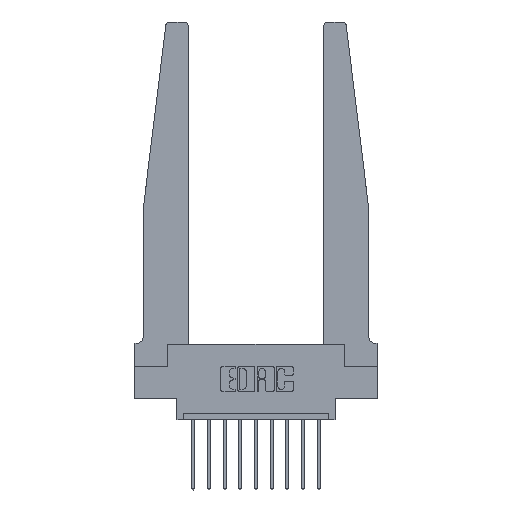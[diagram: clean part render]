
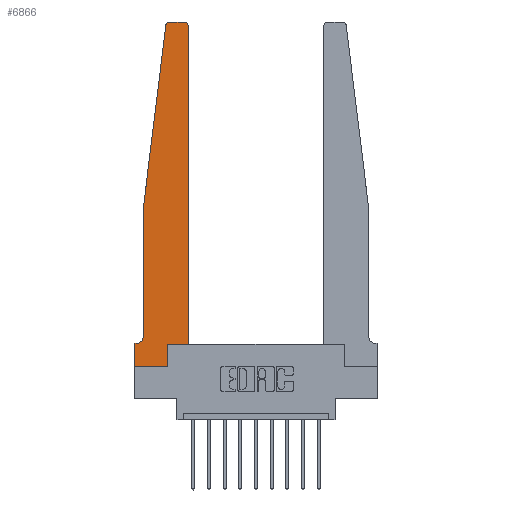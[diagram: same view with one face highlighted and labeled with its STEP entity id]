
A CAD part, top view. The second image highlights one B-rep face of the part: STEP entity #6866.
In plain terms, the highlighted planar face has unit normal (0, 0, 1).
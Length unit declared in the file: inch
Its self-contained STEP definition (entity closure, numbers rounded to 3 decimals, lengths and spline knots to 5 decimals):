
#23 = FACE_OUTER_BOUND ( 'NONE', #9984, .T. ) ;
#167 = VERTEX_POINT ( 'NONE', #3351 ) ;
#314 = DIRECTION ( 'NONE',  ( 0., 0., -1. ) ) ;
#446 = EDGE_CURVE ( 'NONE', #5068, #1741, #1981, .T. ) ;
#472 = DIRECTION ( 'NONE',  ( 0., 0., 1. ) ) ;
#518 = AXIS2_PLACEMENT_3D ( 'NONE', #7931, #11378, #6886 ) ;
#611 = ORIENTED_EDGE ( 'NONE', *, *, #2585, .T. ) ;
#1184 = VECTOR ( 'NONE', #11733, 39.37008 ) ;
#1207 = CARTESIAN_POINT ( 'NONE',  ( 0.425, 2.72, 0.37 ) ) ;
#1356 = AXIS2_PLACEMENT_3D ( 'NONE', #7359, #472, #8464 ) ;
#1529 = EDGE_CURVE ( 'NONE', #8878, #4669, #12413, .T. ) ;
#1741 = VERTEX_POINT ( 'NONE', #7976 ) ;
#1931 = ORIENTED_EDGE ( 'NONE', *, *, #6450, .T. ) ;
#1981 = LINE ( 'NONE', #12524, #12801 ) ;
#1987 = VECTOR ( 'NONE', #13568, 39.37008 ) ;
#2030 = CARTESIAN_POINT ( 'NONE',  ( 0., 0., 0.37 ) ) ;
#2033 = LINE ( 'NONE', #4767, #10503 ) ;
#2230 = CARTESIAN_POINT ( 'NONE',  ( 0., 0., 0.37 ) ) ;
#2353 = DIRECTION ( 'NONE',  ( 1., 0., 0. ) ) ;
#2585 = EDGE_CURVE ( 'NONE', #14409, #12088, #3734, .T. ) ;
#2735 = LINE ( 'NONE', #5553, #1987 ) ;
#2736 = CARTESIAN_POINT ( 'NONE',  ( 0.015, 0.2375, 0.37 ) ) ;
#3072 = LINE ( 'NONE', #10141, #5617 ) ;
#3149 = VERTEX_POINT ( 'NONE', #9297 ) ;
#3351 = CARTESIAN_POINT ( 'NONE',  ( 0.24675, 2.72367, 0.37 ) ) ;
#3624 = DIRECTION ( 'NONE',  ( -1., 0., 0. ) ) ;
#3727 = CIRCLE ( 'NONE', #6720, 0.05 ) ;
#3734 = LINE ( 'NONE', #2030, #5724 ) ;
#3830 = VERTEX_POINT ( 'NONE', #10279 ) ;
#3988 = CIRCLE ( 'NONE', #1356, 0.03 ) ;
#4092 = LINE ( 'NONE', #6100, #1184 ) ;
#4334 = CIRCLE ( 'NONE', #518, 0.03 ) ;
#4591 = DIRECTION ( 'NONE',  ( 0., 0., 1. ) ) ;
#4669 = VERTEX_POINT ( 'NONE', #11202 ) ;
#4767 = CARTESIAN_POINT ( 'NONE',  ( 0.425, 0.18, 0.37 ) ) ;
#5024 = CARTESIAN_POINT ( 'NONE',  ( 0.015, 0.1875, 0.37 ) ) ;
#5068 = VERTEX_POINT ( 'NONE', #6697 ) ;
#5075 = VECTOR ( 'NONE', #6389, 39.37008 ) ;
#5505 = AXIS2_PLACEMENT_3D ( 'NONE', #11585, #4591, #2353 ) ;
#5553 = CARTESIAN_POINT ( 'NONE',  ( 0.065, 1.25, 0.37 ) ) ;
#5617 = VECTOR ( 'NONE', #6676, 39.37008 ) ;
#5724 = VECTOR ( 'NONE', #6767, 39.37008 ) ;
#5848 = ORIENTED_EDGE ( 'NONE', *, *, #8897, .T. ) ;
#6100 = CARTESIAN_POINT ( 'NONE',  ( 0., 0., 0.37 ) ) ;
#6389 = DIRECTION ( 'NONE',  ( 0., -1., 0. ) ) ;
#6450 = EDGE_CURVE ( 'NONE', #3830, #12753, #2033, .T. ) ;
#6676 = DIRECTION ( 'NONE',  ( 0., 1., 0. ) ) ;
#6697 = CARTESIAN_POINT ( 'NONE',  ( 0.395, 2.75, 0.37 ) ) ;
#6720 = AXIS2_PLACEMENT_3D ( 'NONE', #2736, #314, #8323 ) ;
#6765 = EDGE_CURVE ( 'NONE', #12753, #6867, #13022, .T. ) ;
#6767 = DIRECTION ( 'NONE',  ( 1., 0., 0. ) ) ;
#6799 = VERTEX_POINT ( 'NONE', #7937 ) ;
#6801 = ORIENTED_EDGE ( 'NONE', *, *, #8446, .T. ) ;
#6866 = ADVANCED_FACE ( 'NONE', ( #23 ), #10308, .T. ) ;
#6867 = VERTEX_POINT ( 'NONE', #1207 ) ;
#6870 = CARTESIAN_POINT ( 'NONE',  ( 0.2605, 0., 0.37 ) ) ;
#6886 = DIRECTION ( 'NONE',  ( 1., 0., 0. ) ) ;
#7359 = CARTESIAN_POINT ( 'NONE',  ( 0.27653, 2.72, 0.37 ) ) ;
#7384 = LINE ( 'NONE', #11932, #5075 ) ;
#7401 = ORIENTED_EDGE ( 'NONE', *, *, #1529, .T. ) ;
#7629 = ORIENTED_EDGE ( 'NONE', *, *, #13942, .T. ) ;
#7794 = DIRECTION ( 'NONE',  ( 0., 1., 0. ) ) ;
#7931 = CARTESIAN_POINT ( 'NONE',  ( 0.395, 2.72, 0.37 ) ) ;
#7937 = CARTESIAN_POINT ( 'NONE',  ( 0.065, 0.2375, 0.37 ) ) ;
#7948 = EDGE_CURVE ( 'NONE', #167, #3149, #2735, .T. ) ;
#7976 = CARTESIAN_POINT ( 'NONE',  ( 0.27653, 2.75, 0.37 ) ) ;
#8323 = DIRECTION ( 'NONE',  ( -1., 0., 0. ) ) ;
#8404 = ORIENTED_EDGE ( 'NONE', *, *, #6765, .T. ) ;
#8446 = EDGE_CURVE ( 'NONE', #3149, #6799, #7384, .T. ) ;
#8464 = DIRECTION ( 'NONE',  ( 1., 0., 0. ) ) ;
#8559 = EDGE_CURVE ( 'NONE', #12088, #3830, #3072, .T. ) ;
#8878 = VERTEX_POINT ( 'NONE', #5024 ) ;
#8897 = EDGE_CURVE ( 'NONE', #1741, #167, #3988, .T. ) ;
#9029 = DIRECTION ( 'NONE',  ( -1., 0., 0. ) ) ;
#9297 = CARTESIAN_POINT ( 'NONE',  ( 0.065, 1.25, 0.37 ) ) ;
#9299 = CARTESIAN_POINT ( 'NONE',  ( 0.065, 0.1875, 0.37 ) ) ;
#9383 = DIRECTION ( 'NONE',  ( 1., 0., 0. ) ) ;
#9818 = EDGE_CURVE ( 'NONE', #6867, #5068, #4334, .T. ) ;
#9863 = ORIENTED_EDGE ( 'NONE', *, *, #446, .T. ) ;
#9984 = EDGE_LOOP ( 'NONE', ( #9863, #5848, #13586, #6801, #14823, #7401, #7629, #611, #11858, #1931, #8404, #13819 ) ) ;
#10015 = CARTESIAN_POINT ( 'NONE',  ( 0.425, 0.18, 0.37 ) ) ;
#10141 = CARTESIAN_POINT ( 'NONE',  ( 0.2605, 0.18, 0.37 ) ) ;
#10279 = CARTESIAN_POINT ( 'NONE',  ( 0.2605, 0.18, 0.37 ) ) ;
#10308 = PLANE ( 'NONE',  #5505 ) ;
#10503 = VECTOR ( 'NONE', #9383, 39.37008 ) ;
#10967 = VECTOR ( 'NONE', #3624, 39.37008 ) ;
#11202 = CARTESIAN_POINT ( 'NONE',  ( 0., 0.1875, 0.37 ) ) ;
#11378 = DIRECTION ( 'NONE',  ( 0., 0., 1. ) ) ;
#11566 = CARTESIAN_POINT ( 'NONE',  ( 0.425, 0.18, 0.37 ) ) ;
#11585 = CARTESIAN_POINT ( 'NONE',  ( 0., 0.1875, 0.37 ) ) ;
#11733 = DIRECTION ( 'NONE',  ( 0., -1., 0. ) ) ;
#11858 = ORIENTED_EDGE ( 'NONE', *, *, #8559, .T. ) ;
#11932 = CARTESIAN_POINT ( 'NONE',  ( 0.065, 1.25, 0.37 ) ) ;
#12088 = VERTEX_POINT ( 'NONE', #6870 ) ;
#12413 = LINE ( 'NONE', #9299, #10967 ) ;
#12524 = CARTESIAN_POINT ( 'NONE',  ( 0.25, 2.75, 0.37 ) ) ;
#12753 = VERTEX_POINT ( 'NONE', #11566 ) ;
#12801 = VECTOR ( 'NONE', #9029, 39.37008 ) ;
#13022 = LINE ( 'NONE', #10015, #13189 ) ;
#13189 = VECTOR ( 'NONE', #7794, 39.37008 ) ;
#13568 = DIRECTION ( 'NONE',  ( -0.122, -0.992, 0. ) ) ;
#13586 = ORIENTED_EDGE ( 'NONE', *, *, #7948, .T. ) ;
#13819 = ORIENTED_EDGE ( 'NONE', *, *, #9818, .T. ) ;
#13942 = EDGE_CURVE ( 'NONE', #4669, #14409, #4092, .T. ) ;
#14409 = VERTEX_POINT ( 'NONE', #2230 ) ;
#14698 = EDGE_CURVE ( 'NONE', #6799, #8878, #3727, .T. ) ;
#14823 = ORIENTED_EDGE ( 'NONE', *, *, #14698, .T. ) ;
